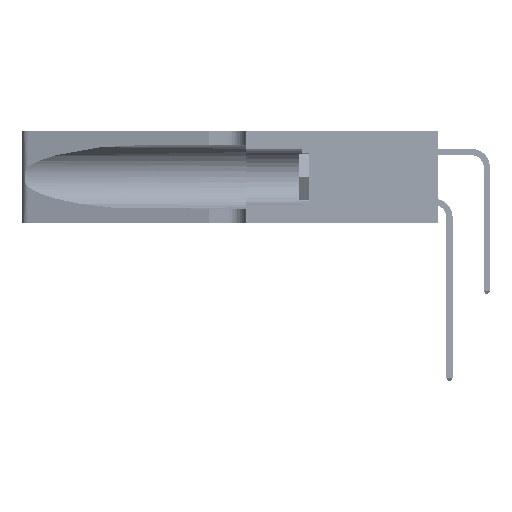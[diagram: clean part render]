
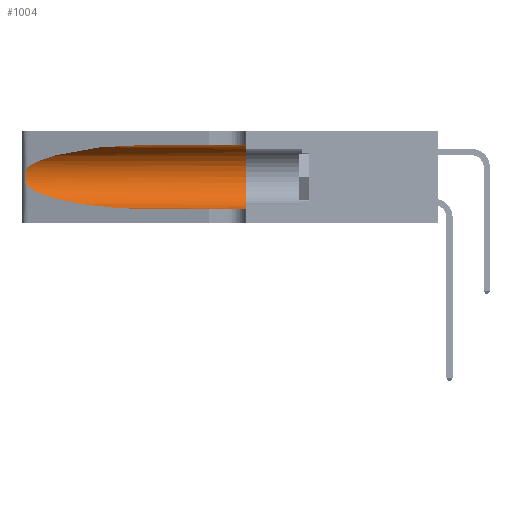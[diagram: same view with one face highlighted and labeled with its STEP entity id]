
A CAD part, left-side view. The second image highlights one B-rep face of the part: STEP entity #1004.
In plain terms, the highlighted cylindrical face has radius 3.308 mm (diameter 6.617 mm), a partial arc.
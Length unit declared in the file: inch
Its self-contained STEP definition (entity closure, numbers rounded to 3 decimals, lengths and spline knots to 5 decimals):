
#355 = CARTESIAN_POINT ( 'NONE',  ( 0.26075, 1.23896, 0.178 ) ) ;
#1004 = ADVANCED_FACE ( 'NONE', ( #23252 ), #12721, .F. ) ;
#1990 =( BOUNDED_CURVE ( )  B_SPLINE_CURVE ( 3, ( #10744, #14371, #18691, #46434 ),
 .UNSPECIFIED., .F., .F. ) 
 B_SPLINE_CURVE_WITH_KNOTS ( ( 4, 4 ),
 ( 3.44316, 4.71239 ),
 .UNSPECIFIED. ) 
 CURVE ( )  GEOMETRIC_REPRESENTATION_ITEM ( )  RATIONAL_B_SPLINE_CURVE ( ( 1., 0.87, 0.87, 1. ) ) 
 REPRESENTATION_ITEM ( '' )  );
#2242 = EDGE_CURVE ( 'NONE', #25807, #17182, #10095, .T. ) ;
#2395 = CARTESIAN_POINT ( 'NONE',  ( 0.25487, 1.22718, 0.14631 ) ) ;
#2980 = DIRECTION ( 'NONE',  ( 0., 1., 0. ) ) ;
#4492 = CARTESIAN_POINT ( 'NONE',  ( 0.25854, 1.2359, 0.20912 ) ) ;
#5727 =( BOUNDED_CURVE ( )  B_SPLINE_CURVE ( 3, ( #30495, #18632, #42912, #10522 ),
 .UNSPECIFIED., .F., .T. ) 
 B_SPLINE_CURVE_WITH_KNOTS ( ( 4, 4 ),
 ( 1.5708, 2.84003 ),
 .UNSPECIFIED. ) 
 CURVE ( )  GEOMETRIC_REPRESENTATION_ITEM ( )  RATIONAL_B_SPLINE_CURVE ( ( 1., 0.87, 0.87, 1. ) ) 
 REPRESENTATION_ITEM ( '' )  );
#7576 = DIRECTION ( 'NONE',  ( 0., 0., -1. ) ) ;
#10095 = CIRCLE ( 'NONE', #26597, 0.13025 ) ;
#10522 = CARTESIAN_POINT ( 'NONE',  ( 0.25487, 1.22718, 0.22369 ) ) ;
#10744 = CARTESIAN_POINT ( 'NONE',  ( 0.25487, 1.22718, 0.14631 ) ) ;
#11704 = CARTESIAN_POINT ( 'NONE',  ( 0.25639, 1.23184, 0.21858 ) ) ;
#11874 = CARTESIAN_POINT ( 'NONE',  ( 0.25856, 1.23593, 0.16098 ) ) ;
#12215 = CARTESIAN_POINT ( 'NONE',  ( 0.25639, 1.23186, 0.15144 ) ) ;
#12284 = CARTESIAN_POINT ( 'NONE',  ( 0.1305, 0.35, 0.31525 ) ) ;
#12532 = VERTEX_POINT ( 'NONE', #30235 ) ;
#12721 = CYLINDRICAL_SURFACE ( 'NONE', #22555, 0.13025 ) ;
#14237 = CARTESIAN_POINT ( 'NONE',  ( 0.1305, 1.61858, 0.31525 ) ) ;
#14371 = CARTESIAN_POINT ( 'NONE',  ( 0.2373, 1.15595, 0.08982 ) ) ;
#15810 = ORIENTED_EDGE ( 'NONE', *, *, #2242, .F. ) ;
#17182 = VERTEX_POINT ( 'NONE', #38435 ) ;
#17286 = ORIENTED_EDGE ( 'NONE', *, *, #45270, .T. ) ;
#17930 = ORIENTED_EDGE ( 'NONE', *, *, #35733, .T. ) ;
#18632 = CARTESIAN_POINT ( 'NONE',  ( 0.18966, 0.96281, 0.31525 ) ) ;
#18691 = CARTESIAN_POINT ( 'NONE',  ( 0.18966, 0.96281, 0.05475 ) ) ;
#18981 = DIRECTION ( 'NONE',  ( 0., -1., 0. ) ) ;
#22195 = DIRECTION ( 'NONE',  ( 0., -1., 0. ) ) ;
#22555 = AXIS2_PLACEMENT_3D ( 'NONE', #31711, #18981, #7576 ) ;
#22953 = VERTEX_POINT ( 'NONE', #46004 ) ;
#23029 = DIRECTION ( 'NONE',  ( 0., -1., 0. ) ) ;
#23252 = FACE_OUTER_BOUND ( 'NONE', #28717, .T. ) ;
#23689 = EDGE_CURVE ( 'NONE', #29256, #22953, #1990, .T. ) ;
#24201 = CARTESIAN_POINT ( 'NONE',  ( 0.25487, 1.22718, 0.22369 ) ) ;
#25584 = ORIENTED_EDGE ( 'NONE', *, *, #30033, .F. ) ;
#25598 = LINE ( 'NONE', #31770, #27419 ) ;
#25807 = VERTEX_POINT ( 'NONE', #12284 ) ;
#26597 = AXIS2_PLACEMENT_3D ( 'NONE', #42800, #2980, #50386 ) ;
#27350 = VECTOR ( 'NONE', #22195, 39.37008 ) ;
#27419 = VECTOR ( 'NONE', #23029, 39.37008 ) ;
#28375 = CARTESIAN_POINT ( 'NONE',  ( 0.26018, 1.23835, 0.19895 ) ) ;
#28717 = EDGE_LOOP ( 'NONE', ( #17286, #17930, #38990, #31377, #15810, #25584 ) ) ;
#29256 = VERTEX_POINT ( 'NONE', #2395 ) ;
#29932 = CARTESIAN_POINT ( 'NONE',  ( 0.1305, 0.72297, 0.31525 ) ) ;
#30033 = EDGE_CURVE ( 'NONE', #38611, #25807, #50288, .T. ) ;
#30235 = CARTESIAN_POINT ( 'NONE',  ( 0.25487, 1.22718, 0.22369 ) ) ;
#30495 = CARTESIAN_POINT ( 'NONE',  ( 0.1305, 0.72297, 0.31525 ) ) ;
#31377 = ORIENTED_EDGE ( 'NONE', *, *, #44594, .T. ) ;
#31711 = CARTESIAN_POINT ( 'NONE',  ( 0.1305, 1.61858, 0.185 ) ) ;
#31770 = CARTESIAN_POINT ( 'NONE',  ( 0.1305, 1.61858, 0.05475 ) ) ;
#31884 = CARTESIAN_POINT ( 'NONE',  ( 0.25487, 1.22718, 0.14631 ) ) ;
#32063 = CARTESIAN_POINT ( 'NONE',  ( 0.25789, 1.23486, 0.15765 ) ) ;
#35697 = CARTESIAN_POINT ( 'NONE',  ( 0.25787, 1.23484, 0.2124 ) ) ;
#35733 = EDGE_CURVE ( 'NONE', #12532, #29256, #50836, .T. ) ;
#35860 = CARTESIAN_POINT ( 'NONE',  ( 0.26075, 1.23896, 0.19203 ) ) ;
#36032 = CARTESIAN_POINT ( 'NONE',  ( 0.26017, 1.23833, 0.17102 ) ) ;
#38435 = CARTESIAN_POINT ( 'NONE',  ( 0.1305, 0.35, 0.05475 ) ) ;
#38611 = VERTEX_POINT ( 'NONE', #29932 ) ;
#38990 = ORIENTED_EDGE ( 'NONE', *, *, #23689, .T. ) ;
#39656 = CARTESIAN_POINT ( 'NONE',  ( 0.25555, 1.22993, 0.14849 ) ) ;
#40170 = CARTESIAN_POINT ( 'NONE',  ( 0.25555, 1.22994, 0.2215 ) ) ;
#42800 = CARTESIAN_POINT ( 'NONE',  ( 0.1305, 0.35, 0.185 ) ) ;
#42912 = CARTESIAN_POINT ( 'NONE',  ( 0.2373, 1.15595, 0.28018 ) ) ;
#44594 = EDGE_CURVE ( 'NONE', #22953, #17182, #25598, .T. ) ;
#45270 = EDGE_CURVE ( 'NONE', #38611, #12532, #5727, .T. ) ;
#46004 = CARTESIAN_POINT ( 'NONE',  ( 0.1305, 0.72297, 0.05475 ) ) ;
#46434 = CARTESIAN_POINT ( 'NONE',  ( 0.1305, 0.72297, 0.05475 ) ) ;
#50288 = LINE ( 'NONE', #14237, #27350 ) ;
#50386 = DIRECTION ( 'NONE',  ( 0., 0., 1. ) ) ;
#50836 = B_SPLINE_CURVE_WITH_KNOTS ( 'NONE', 3,
 ( #24201, #40170, #11704, #35697, #4492, #28375, #35860, #355, #36032, #11874, #32063, #12215, #39656, #31884 ),
 .UNSPECIFIED., .F., .F.,
 ( 4, 2, 2, 2, 2, 2, 4 ),
 ( 0., 0.00027, 0.00053, 0.00107, 0.0016, 0.00187, 0.00214 ),
 .UNSPECIFIED. ) ;
